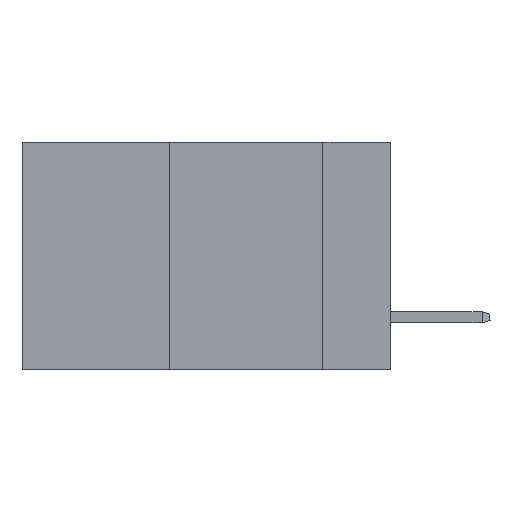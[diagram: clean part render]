
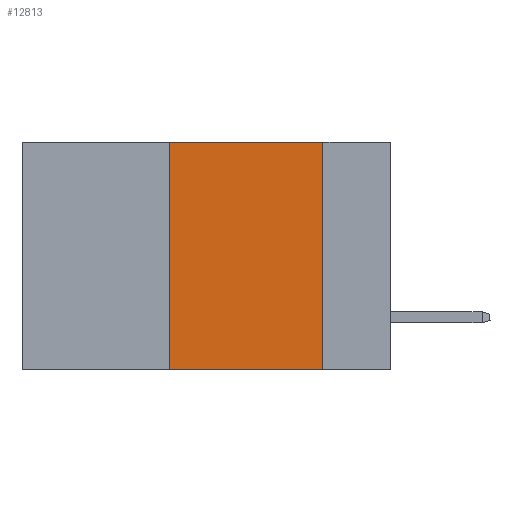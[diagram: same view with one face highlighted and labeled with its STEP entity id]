
A CAD part, left-side view. The second image highlights one B-rep face of the part: STEP entity #12813.
In plain terms, the highlighted planar face has unit normal (-1, 0, 0).
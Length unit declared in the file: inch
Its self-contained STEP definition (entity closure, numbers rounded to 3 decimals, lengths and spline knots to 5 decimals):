
#541 = LINE ( 'NONE', #15804, #11040 ) ;
#962 = DIRECTION ( 'NONE',  ( 0., 0., 1. ) ) ;
#2925 = LINE ( 'NONE', #16575, #10855 ) ;
#3627 = VECTOR ( 'NONE', #13671, 39.37008 ) ;
#3671 = CARTESIAN_POINT ( 'NONE',  ( 0., 0.36, 0. ) ) ;
#4180 = ORIENTED_EDGE ( 'NONE', *, *, #10827, .F. ) ;
#6202 = PLANE ( 'NONE',  #16640 ) ;
#6563 = FACE_OUTER_BOUND ( 'NONE', #6569, .T. ) ;
#6569 = EDGE_LOOP ( 'NONE', ( #21234, #17856, #4180, #16072 ) ) ;
#8640 = EDGE_CURVE ( 'NONE', #15330, #16668, #2925, .T. ) ;
#9663 = DIRECTION ( 'NONE',  ( 0., 0., -1. ) ) ;
#9801 = EDGE_CURVE ( 'NONE', #15194, #15330, #14152, .T. ) ;
#10155 = CARTESIAN_POINT ( 'NONE',  ( 0., 0.11, -0.37 ) ) ;
#10372 = CARTESIAN_POINT ( 'NONE',  ( 0., 0.6, 0. ) ) ;
#10827 = EDGE_CURVE ( 'NONE', #11677, #15194, #541, .T. ) ;
#10855 = VECTOR ( 'NONE', #9663, 39.37008 ) ;
#11040 = VECTOR ( 'NONE', #962, 39.37008 ) ;
#11409 = DIRECTION ( 'NONE',  ( 0., 0., -1. ) ) ;
#11671 = CARTESIAN_POINT ( 'NONE',  ( 0., 0.36, -0.37 ) ) ;
#11677 = VERTEX_POINT ( 'NONE', #11671 ) ;
#12813 = ADVANCED_FACE ( 'NONE', ( #6563 ), #6202, .F. ) ;
#13096 = VECTOR ( 'NONE', #18284, 39.37008 ) ;
#13627 = LINE ( 'NONE', #16622, #13096 ) ;
#13671 = DIRECTION ( 'NONE',  ( 0., -1., 0. ) ) ;
#14152 = LINE ( 'NONE', #10372, #3627 ) ;
#14483 = DIRECTION ( 'NONE',  ( 1., 0., 0. ) ) ;
#15194 = VERTEX_POINT ( 'NONE', #3671 ) ;
#15330 = VERTEX_POINT ( 'NONE', #20349 ) ;
#15804 = CARTESIAN_POINT ( 'NONE',  ( 0., 0.36, 0. ) ) ;
#16072 = ORIENTED_EDGE ( 'NONE', *, *, #20176, .T. ) ;
#16401 = CARTESIAN_POINT ( 'NONE',  ( 0., 0.6, 0. ) ) ;
#16575 = CARTESIAN_POINT ( 'NONE',  ( 0., 0.11, 0. ) ) ;
#16622 = CARTESIAN_POINT ( 'NONE',  ( 0., 0.6, -0.37 ) ) ;
#16640 = AXIS2_PLACEMENT_3D ( 'NONE', #16401, #14483, #11409 ) ;
#16668 = VERTEX_POINT ( 'NONE', #10155 ) ;
#17856 = ORIENTED_EDGE ( 'NONE', *, *, #9801, .F. ) ;
#18284 = DIRECTION ( 'NONE',  ( 0., -1., 0. ) ) ;
#20176 = EDGE_CURVE ( 'NONE', #11677, #16668, #13627, .T. ) ;
#20349 = CARTESIAN_POINT ( 'NONE',  ( 0., 0.11, 0. ) ) ;
#21234 = ORIENTED_EDGE ( 'NONE', *, *, #8640, .F. ) ;
